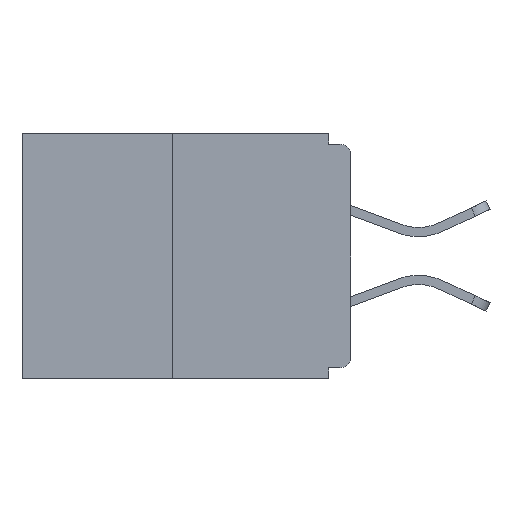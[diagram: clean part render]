
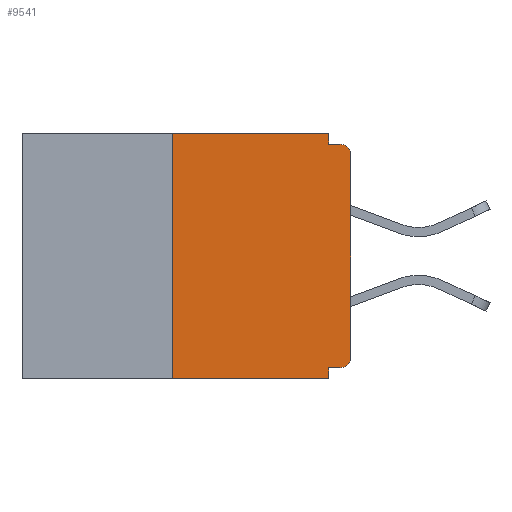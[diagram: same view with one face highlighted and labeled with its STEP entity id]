
A CAD part, left-side view. The second image highlights one B-rep face of the part: STEP entity #9541.
In plain terms, the highlighted planar face has unit normal (-1, 0, 0).
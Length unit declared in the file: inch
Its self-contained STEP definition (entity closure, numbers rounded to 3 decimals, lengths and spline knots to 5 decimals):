
#135 = CARTESIAN_POINT ( 'NONE',  ( 0., 0.46, -0.343 ) ) ;
#299 = CARTESIAN_POINT ( 'NONE',  ( 0., 0.031, -0.015 ) ) ;
#547 = EDGE_CURVE ( 'NONE', #1143, #14583, #14561, .T. ) ;
#693 = ORIENTED_EDGE ( 'NONE', *, *, #547, .T. ) ;
#982 = CARTESIAN_POINT ( 'NONE',  ( 0., 0., -0.313 ) ) ;
#1143 = VERTEX_POINT ( 'NONE', #10745 ) ;
#1301 = AXIS2_PLACEMENT_3D ( 'NONE', #21543, #12106, #19576 ) ;
#1898 = DIRECTION ( 'NONE',  ( -1., 0., 0. ) ) ;
#1985 = EDGE_CURVE ( 'NONE', #6739, #13540, #16154, .T. ) ;
#2195 = EDGE_CURVE ( 'NONE', #8362, #14583, #17651, .T. ) ;
#2228 = ORIENTED_EDGE ( 'NONE', *, *, #2195, .F. ) ;
#2413 = EDGE_LOOP ( 'NONE', ( #20859, #2979, #13183, #8021, #13572, #11660, #14930, #693, #2228, #14786 ) ) ;
#2951 = CARTESIAN_POINT ( 'NONE',  ( 0., 0.031, 0. ) ) ;
#2979 = ORIENTED_EDGE ( 'NONE', *, *, #17669, .F. ) ;
#3023 = CARTESIAN_POINT ( 'NONE',  ( 0., 0.015, -0.328 ) ) ;
#3065 = DIRECTION ( 'NONE',  ( 0., 0., -1. ) ) ;
#3475 = CARTESIAN_POINT ( 'NONE',  ( 0., 0.015, -0.313 ) ) ;
#4657 = DIRECTION ( 'NONE',  ( 0., 0., 1. ) ) ;
#4846 = CARTESIAN_POINT ( 'NONE',  ( 0., 0.031, -0.343 ) ) ;
#5005 = LINE ( 'NONE', #20675, #6268 ) ;
#5300 = DIRECTION ( 'NONE',  ( 0., 1., 0. ) ) ;
#5390 = DIRECTION ( 'NONE',  ( 0., -1., 0. ) ) ;
#5644 = LINE ( 'NONE', #21190, #11941 ) ;
#6024 = EDGE_CURVE ( 'NONE', #10381, #6257, #9251, .T. ) ;
#6257 = VERTEX_POINT ( 'NONE', #7834 ) ;
#6268 = VECTOR ( 'NONE', #18943, 39.37008 ) ;
#6288 = CIRCLE ( 'NONE', #14890, 0.015 ) ;
#6739 = VERTEX_POINT ( 'NONE', #16468 ) ;
#7126 = VERTEX_POINT ( 'NONE', #982 ) ;
#7787 = VERTEX_POINT ( 'NONE', #9845 ) ;
#7834 = CARTESIAN_POINT ( 'NONE',  ( 0., 0.031, 0. ) ) ;
#8021 = ORIENTED_EDGE ( 'NONE', *, *, #19974, .F. ) ;
#8362 = VERTEX_POINT ( 'NONE', #299 ) ;
#8769 = DIRECTION ( 'NONE',  ( 0., -1., 0. ) ) ;
#8895 = CARTESIAN_POINT ( 'NONE',  ( 0., 0.015, -0.015 ) ) ;
#9028 = VECTOR ( 'NONE', #18024, 39.37008 ) ;
#9251 = LINE ( 'NONE', #21288, #12871 ) ;
#9541 = ADVANCED_FACE ( 'NONE', ( #10591 ), #12452, .F. ) ;
#9845 = CARTESIAN_POINT ( 'NONE',  ( 0., 0.031, -0.328 ) ) ;
#10381 = VERTEX_POINT ( 'NONE', #19995 ) ;
#10554 = EDGE_CURVE ( 'NONE', #6257, #8362, #13334, .T. ) ;
#10591 = FACE_OUTER_BOUND ( 'NONE', #2413, .T. ) ;
#10745 = CARTESIAN_POINT ( 'NONE',  ( 0., 0., -0.03 ) ) ;
#11597 = EDGE_CURVE ( 'NONE', #18860, #7787, #5644, .T. ) ;
#11660 = ORIENTED_EDGE ( 'NONE', *, *, #16515, .T. ) ;
#11941 = VECTOR ( 'NONE', #5300, 39.37008 ) ;
#12106 = DIRECTION ( 'NONE',  ( 1., 0., 0. ) ) ;
#12111 = DIRECTION ( 'NONE',  ( 0., 0., -1. ) ) ;
#12169 = CARTESIAN_POINT ( 'NONE',  ( 0., 0.015, -0.03 ) ) ;
#12452 = PLANE ( 'NONE',  #1301 ) ;
#12871 = VECTOR ( 'NONE', #5390, 39.37008 ) ;
#13183 = ORIENTED_EDGE ( 'NONE', *, *, #1985, .T. ) ;
#13187 = CARTESIAN_POINT ( 'NONE',  ( 0., 0.25, 0. ) ) ;
#13334 = LINE ( 'NONE', #2951, #13895 ) ;
#13540 = VERTEX_POINT ( 'NONE', #20605 ) ;
#13572 = ORIENTED_EDGE ( 'NONE', *, *, #11597, .F. ) ;
#13787 = VECTOR ( 'NONE', #12111, 39.37008 ) ;
#13895 = VECTOR ( 'NONE', #3065, 39.37008 ) ;
#13905 = CARTESIAN_POINT ( 'NONE',  ( 0., 0., -0.015 ) ) ;
#14341 = DIRECTION ( 'NONE',  ( 0., 0., -1. ) ) ;
#14561 = CIRCLE ( 'NONE', #17555, 0.015 ) ;
#14583 = VERTEX_POINT ( 'NONE', #8895 ) ;
#14786 = ORIENTED_EDGE ( 'NONE', *, *, #10554, .F. ) ;
#14890 = AXIS2_PLACEMENT_3D ( 'NONE', #3475, #21226, #14341 ) ;
#14930 = ORIENTED_EDGE ( 'NONE', *, *, #18421, .T. ) ;
#14963 = LINE ( 'NONE', #13187, #21174 ) ;
#16034 = DIRECTION ( 'NONE',  ( 0., 0., -1. ) ) ;
#16154 = LINE ( 'NONE', #135, #9028 ) ;
#16468 = CARTESIAN_POINT ( 'NONE',  ( 0., 0.25, -0.343 ) ) ;
#16515 = EDGE_CURVE ( 'NONE', #18860, #7126, #6288, .T. ) ;
#17555 = AXIS2_PLACEMENT_3D ( 'NONE', #12169, #1898, #16034 ) ;
#17651 = LINE ( 'NONE', #13905, #22822 ) ;
#17669 = EDGE_CURVE ( 'NONE', #6739, #10381, #14963, .T. ) ;
#18024 = DIRECTION ( 'NONE',  ( 0., -1., 0. ) ) ;
#18421 = EDGE_CURVE ( 'NONE', #7126, #1143, #5005, .T. ) ;
#18860 = VERTEX_POINT ( 'NONE', #3023 ) ;
#18943 = DIRECTION ( 'NONE',  ( 0., 0., 1. ) ) ;
#19576 = DIRECTION ( 'NONE',  ( 0., 0., -1. ) ) ;
#19974 = EDGE_CURVE ( 'NONE', #7787, #13540, #22601, .T. ) ;
#19995 = CARTESIAN_POINT ( 'NONE',  ( 0., 0.25, 0. ) ) ;
#20605 = CARTESIAN_POINT ( 'NONE',  ( 0., 0.031, -0.343 ) ) ;
#20675 = CARTESIAN_POINT ( 'NONE',  ( 0., 0., 0. ) ) ;
#20859 = ORIENTED_EDGE ( 'NONE', *, *, #6024, .F. ) ;
#21174 = VECTOR ( 'NONE', #4657, 39.37008 ) ;
#21190 = CARTESIAN_POINT ( 'NONE',  ( 0., 0., -0.328 ) ) ;
#21226 = DIRECTION ( 'NONE',  ( -1., 0., 0. ) ) ;
#21288 = CARTESIAN_POINT ( 'NONE',  ( 0., 0.46, 0. ) ) ;
#21543 = CARTESIAN_POINT ( 'NONE',  ( 0., 0.46, 0. ) ) ;
#22601 = LINE ( 'NONE', #4846, #13787 ) ;
#22822 = VECTOR ( 'NONE', #8769, 39.37008 ) ;
